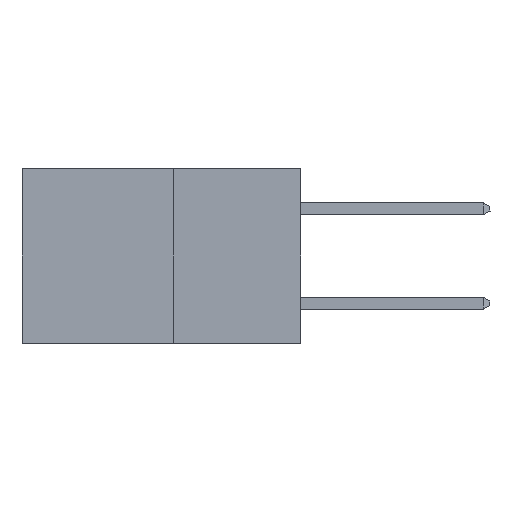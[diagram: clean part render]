
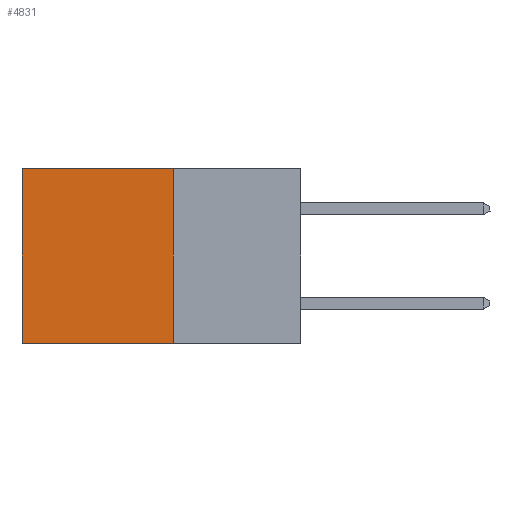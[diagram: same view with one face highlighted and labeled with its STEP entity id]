
A CAD part, left-side view. The second image highlights one B-rep face of the part: STEP entity #4831.
In plain terms, the highlighted planar face has unit normal (-1, 0, 0).
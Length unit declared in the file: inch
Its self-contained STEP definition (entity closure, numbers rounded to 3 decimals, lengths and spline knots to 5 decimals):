
#262 = CARTESIAN_POINT ( 'NONE',  ( 0.277, 0.59, -0.37 ) ) ;
#936 = AXIS2_PLACEMENT_3D ( 'NONE', #5812, #5376, #4927 ) ;
#1161 = VERTEX_POINT ( 'NONE', #7388 ) ;
#1270 = FACE_OUTER_BOUND ( 'NONE', #7781, .T. ) ;
#1298 = ORIENTED_EDGE ( 'NONE', *, *, #6540, .F. ) ;
#1450 = PLANE ( 'NONE',  #936 ) ;
#2222 = ORIENTED_EDGE ( 'NONE', *, *, #2828, .F. ) ;
#2290 = VERTEX_POINT ( 'NONE', #262 ) ;
#2457 = ORIENTED_EDGE ( 'NONE', *, *, #6028, .T. ) ;
#2596 = CARTESIAN_POINT ( 'NONE',  ( 0.277, 0.59, -0.37 ) ) ;
#2769 = LINE ( 'NONE', #5163, #4388 ) ;
#2828 = EDGE_CURVE ( 'NONE', #1161, #4618, #4496, .T. ) ;
#2908 = CARTESIAN_POINT ( 'NONE',  ( 0.277, 0.27, -0.37 ) ) ;
#3089 = ORIENTED_EDGE ( 'NONE', *, *, #5656, .T. ) ;
#3099 = VECTOR ( 'NONE', #5047, 39.37008 ) ;
#3248 = LINE ( 'NONE', #2596, #6480 ) ;
#3380 = DIRECTION ( 'NONE',  ( 0., 1., 0. ) ) ;
#4019 = LINE ( 'NONE', #6209, #5397 ) ;
#4388 = VECTOR ( 'NONE', #3380, 39.37008 ) ;
#4496 = LINE ( 'NONE', #5070, #3099 ) ;
#4618 = VERTEX_POINT ( 'NONE', #2908 ) ;
#4831 = ADVANCED_FACE ( 'NONE', ( #1270 ), #1450, .F. ) ;
#4927 = DIRECTION ( 'NONE',  ( 0., 0., -1. ) ) ;
#5047 = DIRECTION ( 'NONE',  ( 0., 0., -1. ) ) ;
#5070 = CARTESIAN_POINT ( 'NONE',  ( 0.277, 0.27, -0.37 ) ) ;
#5163 = CARTESIAN_POINT ( 'NONE',  ( 0.277, 0.27, -0.37 ) ) ;
#5376 = DIRECTION ( 'NONE',  ( 1., 0., 0. ) ) ;
#5397 = VECTOR ( 'NONE', #5619, 39.37008 ) ;
#5619 = DIRECTION ( 'NONE',  ( 0., 1., 0. ) ) ;
#5656 = EDGE_CURVE ( 'NONE', #7125, #2290, #3248, .T. ) ;
#5812 = CARTESIAN_POINT ( 'NONE',  ( 0.277, 0.27, -0.37 ) ) ;
#5849 = DIRECTION ( 'NONE',  ( 0., 0., -1. ) ) ;
#6028 = EDGE_CURVE ( 'NONE', #1161, #7125, #4019, .T. ) ;
#6209 = CARTESIAN_POINT ( 'NONE',  ( 0.277, 0.27, 0. ) ) ;
#6480 = VECTOR ( 'NONE', #5849, 39.37008 ) ;
#6540 = EDGE_CURVE ( 'NONE', #4618, #2290, #2769, .T. ) ;
#7125 = VERTEX_POINT ( 'NONE', #7220 ) ;
#7220 = CARTESIAN_POINT ( 'NONE',  ( 0.277, 0.59, 0. ) ) ;
#7388 = CARTESIAN_POINT ( 'NONE',  ( 0.277, 0.27, 0. ) ) ;
#7781 = EDGE_LOOP ( 'NONE', ( #3089, #1298, #2222, #2457 ) ) ;
